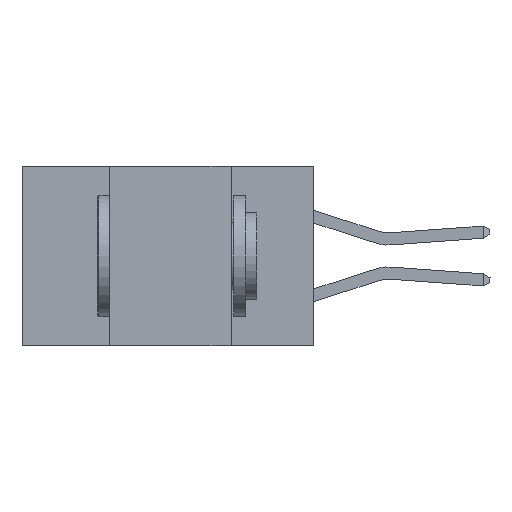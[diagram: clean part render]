
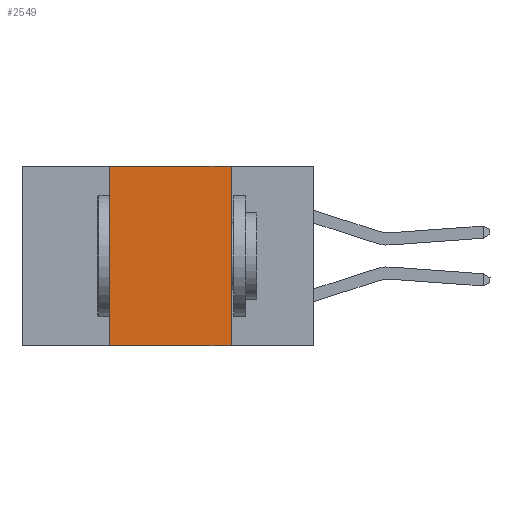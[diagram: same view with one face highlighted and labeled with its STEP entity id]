
A CAD part, left-side view. The second image highlights one B-rep face of the part: STEP entity #2549.
In plain terms, the highlighted planar face has unit normal (-1, 0, 0).
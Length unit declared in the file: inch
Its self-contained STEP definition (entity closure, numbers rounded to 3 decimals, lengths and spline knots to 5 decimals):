
#394 = LINE ( 'NONE', #20249, #4565 ) ;
#913 = AXIS2_PLACEMENT_3D ( 'NONE', #5320, #5275, #5252 ) ;
#2411 = CARTESIAN_POINT ( 'NONE',  ( 0., 0.42, 0. ) ) ;
#2549 = ADVANCED_FACE ( 'NONE', ( #21176 ), #5565, .F. ) ;
#3357 = EDGE_LOOP ( 'NONE', ( #11983, #8417, #5968, #7070 ) ) ;
#4147 = VECTOR ( 'NONE', #12702, 39.37008 ) ;
#4565 = VECTOR ( 'NONE', #11552, 39.37008 ) ;
#4826 = VECTOR ( 'NONE', #21759, 39.37008 ) ;
#5252 = DIRECTION ( 'NONE',  ( 0., 0., -1. ) ) ;
#5275 = DIRECTION ( 'NONE',  ( 1., 0., 0. ) ) ;
#5320 = CARTESIAN_POINT ( 'NONE',  ( 0., 0.6, 0. ) ) ;
#5565 = PLANE ( 'NONE',  #913 ) ;
#5817 = EDGE_CURVE ( 'NONE', #22125, #20794, #18380, .T. ) ;
#5953 = CARTESIAN_POINT ( 'NONE',  ( 0., 0.17, -0.37 ) ) ;
#5968 = ORIENTED_EDGE ( 'NONE', *, *, #5817, .F. ) ;
#7070 = ORIENTED_EDGE ( 'NONE', *, *, #10644, .T. ) ;
#7851 = EDGE_CURVE ( 'NONE', #7920, #21336, #394, .T. ) ;
#7920 = VERTEX_POINT ( 'NONE', #22184 ) ;
#8083 = DIRECTION ( 'NONE',  ( 0., 0., 1. ) ) ;
#8417 = ORIENTED_EDGE ( 'NONE', *, *, #15087, .F. ) ;
#10644 = EDGE_CURVE ( 'NONE', #22125, #21336, #14024, .T. ) ;
#11552 = DIRECTION ( 'NONE',  ( 0., 0., -1. ) ) ;
#11983 = ORIENTED_EDGE ( 'NONE', *, *, #7851, .F. ) ;
#12702 = DIRECTION ( 'NONE',  ( 0., -1., 0. ) ) ;
#13710 = VECTOR ( 'NONE', #8083, 39.37008 ) ;
#14024 = LINE ( 'NONE', #21357, #4147 ) ;
#14672 = LINE ( 'NONE', #18344, #4826 ) ;
#15074 = CARTESIAN_POINT ( 'NONE',  ( 0., 0.42, 0. ) ) ;
#15087 = EDGE_CURVE ( 'NONE', #20794, #7920, #14672, .T. ) ;
#18344 = CARTESIAN_POINT ( 'NONE',  ( 0., 0.6, 0. ) ) ;
#18380 = LINE ( 'NONE', #15074, #13710 ) ;
#20249 = CARTESIAN_POINT ( 'NONE',  ( 0., 0.17, 0. ) ) ;
#20538 = CARTESIAN_POINT ( 'NONE',  ( 0., 0.42, -0.37 ) ) ;
#20794 = VERTEX_POINT ( 'NONE', #2411 ) ;
#21176 = FACE_OUTER_BOUND ( 'NONE', #3357, .T. ) ;
#21336 = VERTEX_POINT ( 'NONE', #5953 ) ;
#21357 = CARTESIAN_POINT ( 'NONE',  ( 0., 0.6, -0.37 ) ) ;
#21759 = DIRECTION ( 'NONE',  ( 0., -1., 0. ) ) ;
#22125 = VERTEX_POINT ( 'NONE', #20538 ) ;
#22184 = CARTESIAN_POINT ( 'NONE',  ( 0., 0.17, 0. ) ) ;
